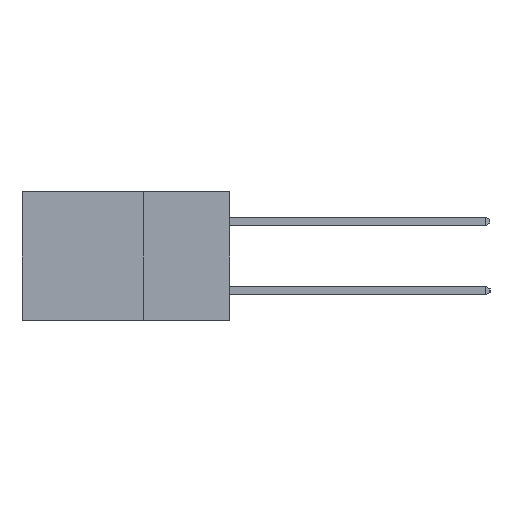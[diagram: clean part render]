
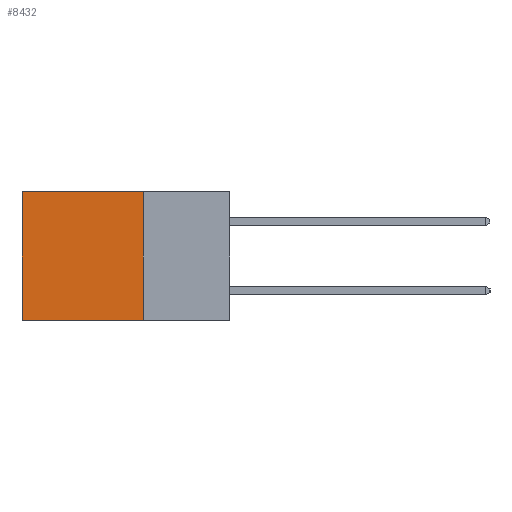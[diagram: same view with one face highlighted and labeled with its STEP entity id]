
A CAD part, left-side view. The second image highlights one B-rep face of the part: STEP entity #8432.
In plain terms, the highlighted planar face has unit normal (-1, 0, 0).
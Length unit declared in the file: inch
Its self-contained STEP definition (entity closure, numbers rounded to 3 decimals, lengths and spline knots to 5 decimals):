
#30 = CARTESIAN_POINT ( 'NONE',  ( 0.2615, 0.25, -0.37 ) ) ;
#231 = EDGE_CURVE ( 'NONE', #3870, #9611, #12829, .T. ) ;
#608 = CARTESIAN_POINT ( 'NONE',  ( 0.2615, 0.25, -0.37 ) ) ;
#866 = DIRECTION ( 'NONE',  ( 0., 1., 0. ) ) ;
#1306 = DIRECTION ( 'NONE',  ( 1., 0., 0. ) ) ;
#1787 = DIRECTION ( 'NONE',  ( 0., 0., -1. ) ) ;
#2013 = VERTEX_POINT ( 'NONE', #11679 ) ;
#3870 = VERTEX_POINT ( 'NONE', #3950 ) ;
#3950 = CARTESIAN_POINT ( 'NONE',  ( 0.2615, 0.6, 0. ) ) ;
#4127 = VECTOR ( 'NONE', #15861, 39.37008 ) ;
#4710 = LINE ( 'NONE', #13615, #10734 ) ;
#5385 = ORIENTED_EDGE ( 'NONE', *, *, #11942, .F. ) ;
#5401 = CARTESIAN_POINT ( 'NONE',  ( 0.2615, 0.6, -0.37 ) ) ;
#7258 = AXIS2_PLACEMENT_3D ( 'NONE', #30, #1306, #10244 ) ;
#7541 = LINE ( 'NONE', #8280, #4127 ) ;
#8069 = FACE_OUTER_BOUND ( 'NONE', #14124, .T. ) ;
#8280 = CARTESIAN_POINT ( 'NONE',  ( 0.2615, 0.25, 0. ) ) ;
#8382 = ORIENTED_EDGE ( 'NONE', *, *, #9467, .F. ) ;
#8432 = ADVANCED_FACE ( 'NONE', ( #8069 ), #15247, .F. ) ;
#8642 = VECTOR ( 'NONE', #1787, 39.37008 ) ;
#8884 = ORIENTED_EDGE ( 'NONE', *, *, #231, .T. ) ;
#9041 = LINE ( 'NONE', #608, #8642 ) ;
#9467 = EDGE_CURVE ( 'NONE', #2013, #11438, #9041, .T. ) ;
#9611 = VERTEX_POINT ( 'NONE', #13586 ) ;
#10244 = DIRECTION ( 'NONE',  ( 0., 0., -1. ) ) ;
#10352 = ORIENTED_EDGE ( 'NONE', *, *, #11279, .T. ) ;
#10734 = VECTOR ( 'NONE', #866, 39.37008 ) ;
#11279 = EDGE_CURVE ( 'NONE', #2013, #3870, #7541, .T. ) ;
#11438 = VERTEX_POINT ( 'NONE', #11440 ) ;
#11440 = CARTESIAN_POINT ( 'NONE',  ( 0.2615, 0.25, -0.37 ) ) ;
#11679 = CARTESIAN_POINT ( 'NONE',  ( 0.2615, 0.25, 0. ) ) ;
#11942 = EDGE_CURVE ( 'NONE', #11438, #9611, #4710, .T. ) ;
#12442 = VECTOR ( 'NONE', #13202, 39.37008 ) ;
#12829 = LINE ( 'NONE', #5401, #12442 ) ;
#13202 = DIRECTION ( 'NONE',  ( 0., 0., -1. ) ) ;
#13586 = CARTESIAN_POINT ( 'NONE',  ( 0.2615, 0.6, -0.37 ) ) ;
#13615 = CARTESIAN_POINT ( 'NONE',  ( 0.2615, 0.25, -0.37 ) ) ;
#14124 = EDGE_LOOP ( 'NONE', ( #8884, #5385, #8382, #10352 ) ) ;
#15247 = PLANE ( 'NONE',  #7258 ) ;
#15861 = DIRECTION ( 'NONE',  ( 0., 1., 0. ) ) ;
